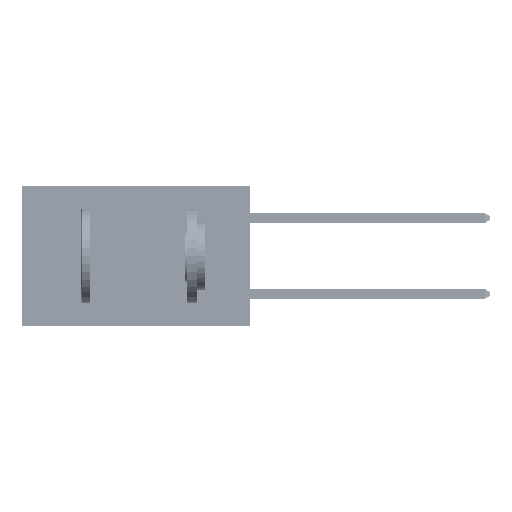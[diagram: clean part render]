
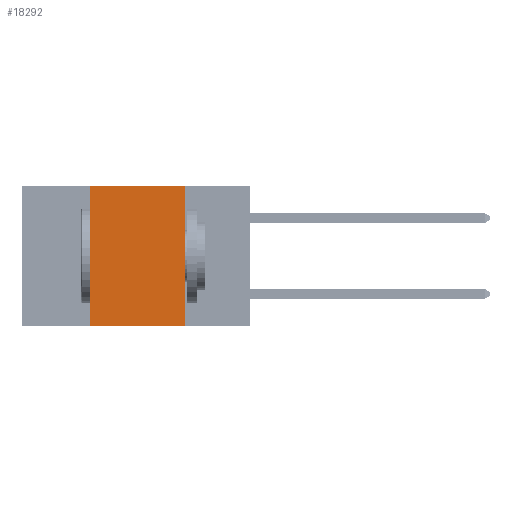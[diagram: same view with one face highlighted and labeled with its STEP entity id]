
A CAD part, left-side view. The second image highlights one B-rep face of the part: STEP entity #18292.
In plain terms, the highlighted planar face has unit normal (-1, 0, 0).
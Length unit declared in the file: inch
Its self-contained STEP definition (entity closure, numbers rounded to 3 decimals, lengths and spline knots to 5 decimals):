
#2846 = ORIENTED_EDGE ( 'NONE', *, *, #11986, .F. ) ;
#3083 = EDGE_CURVE ( 'NONE', #24224, #19964, #23165, .T. ) ;
#4511 = VERTEX_POINT ( 'NONE', #31952 ) ;
#6006 = FACE_OUTER_BOUND ( 'NONE', #24700, .T. ) ;
#8168 = VERTEX_POINT ( 'NONE', #45183 ) ;
#8491 = AXIS2_PLACEMENT_3D ( 'NONE', #40925, #21984, #48325 ) ;
#10548 = VECTOR ( 'NONE', #39747, 39.37008 ) ;
#11006 = ORIENTED_EDGE ( 'NONE', *, *, #23928, .F. ) ;
#11278 = CARTESIAN_POINT ( 'NONE',  ( 0., 0.6, -0.37 ) ) ;
#11986 = EDGE_CURVE ( 'NONE', #19964, #8168, #24296, .T. ) ;
#16133 = DIRECTION ( 'NONE',  ( 0., -1., 0. ) ) ;
#16431 = LINE ( 'NONE', #17642, #10548 ) ;
#17642 = CARTESIAN_POINT ( 'NONE',  ( 0., 0.42, 0. ) ) ;
#18292 = ADVANCED_FACE ( 'NONE', ( #6006 ), #18344, .F. ) ;
#18344 = PLANE ( 'NONE',  #8491 ) ;
#19964 = VERTEX_POINT ( 'NONE', #32933 ) ;
#20283 = VECTOR ( 'NONE', #33197, 39.37008 ) ;
#20786 = ORIENTED_EDGE ( 'NONE', *, *, #3083, .F. ) ;
#21984 = DIRECTION ( 'NONE',  ( 1., 0., 0. ) ) ;
#23165 = LINE ( 'NONE', #38384, #36758 ) ;
#23604 = DIRECTION ( 'NONE',  ( 0., 0., -1. ) ) ;
#23928 = EDGE_CURVE ( 'NONE', #4511, #24224, #16431, .T. ) ;
#24224 = VERTEX_POINT ( 'NONE', #33806 ) ;
#24296 = LINE ( 'NONE', #42711, #36068 ) ;
#24700 = EDGE_LOOP ( 'NONE', ( #2846, #20786, #11006, #34253 ) ) ;
#31952 = CARTESIAN_POINT ( 'NONE',  ( 0., 0.42, -0.37 ) ) ;
#32933 = CARTESIAN_POINT ( 'NONE',  ( 0., 0.17, 0. ) ) ;
#33197 = DIRECTION ( 'NONE',  ( 0., -1., 0. ) ) ;
#33806 = CARTESIAN_POINT ( 'NONE',  ( 0., 0.42, 0. ) ) ;
#34253 = ORIENTED_EDGE ( 'NONE', *, *, #46544, .T. ) ;
#36068 = VECTOR ( 'NONE', #23604, 39.37008 ) ;
#36758 = VECTOR ( 'NONE', #16133, 39.37008 ) ;
#38384 = CARTESIAN_POINT ( 'NONE',  ( 0., 0.6, 0. ) ) ;
#39747 = DIRECTION ( 'NONE',  ( 0., 0., 1. ) ) ;
#40925 = CARTESIAN_POINT ( 'NONE',  ( 0., 0.6, 0. ) ) ;
#42691 = LINE ( 'NONE', #11278, #20283 ) ;
#42711 = CARTESIAN_POINT ( 'NONE',  ( 0., 0.17, 0. ) ) ;
#45183 = CARTESIAN_POINT ( 'NONE',  ( 0., 0.17, -0.37 ) ) ;
#46544 = EDGE_CURVE ( 'NONE', #4511, #8168, #42691, .T. ) ;
#48325 = DIRECTION ( 'NONE',  ( 0., 0., -1. ) ) ;
